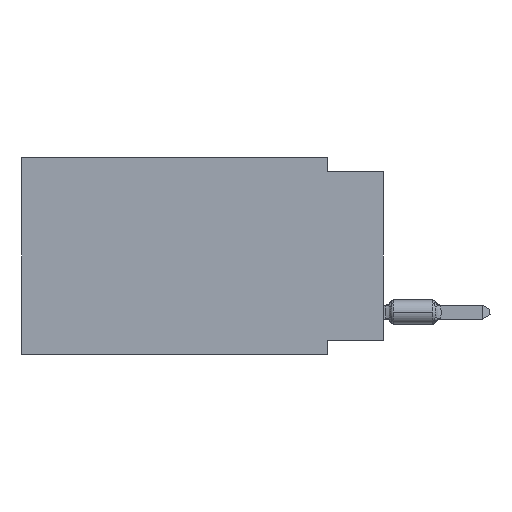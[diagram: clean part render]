
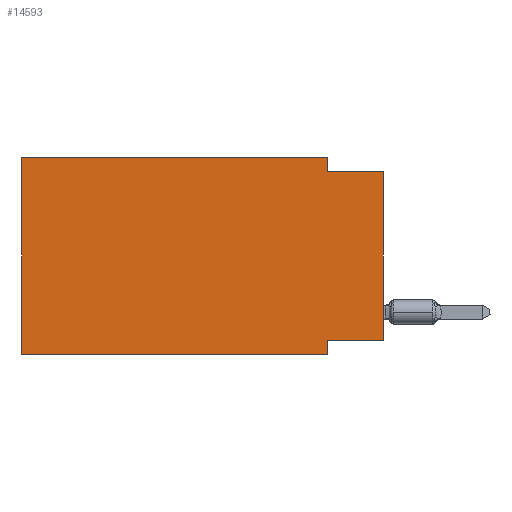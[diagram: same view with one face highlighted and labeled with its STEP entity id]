
A CAD part, left-side view. The second image highlights one B-rep face of the part: STEP entity #14593.
In plain terms, the highlighted planar face has unit normal (-1, 0, 0).
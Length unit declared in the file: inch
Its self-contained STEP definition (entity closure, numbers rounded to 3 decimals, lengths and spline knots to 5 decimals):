
#57 = LINE ( 'NONE', #17755, #11710 ) ;
#176 = CARTESIAN_POINT ( 'NONE',  ( 0., 0., -0.025 ) ) ;
#283 = LINE ( 'NONE', #176, #20078 ) ;
#619 = VERTEX_POINT ( 'NONE', #20172 ) ;
#1433 = EDGE_CURVE ( 'NONE', #3053, #3446, #9642, .T. ) ;
#1984 = CARTESIAN_POINT ( 'NONE',  ( 0., 0.645, 0. ) ) ;
#2115 = VECTOR ( 'NONE', #2336, 39.37008 ) ;
#2336 = DIRECTION ( 'NONE',  ( 0., 1., 0. ) ) ;
#2462 = VERTEX_POINT ( 'NONE', #4624 ) ;
#2981 = DIRECTION ( 'NONE',  ( 0., -1., 0. ) ) ;
#3053 = VERTEX_POINT ( 'NONE', #13976 ) ;
#3055 = LINE ( 'NONE', #16141, #8898 ) ;
#3446 = VERTEX_POINT ( 'NONE', #13425 ) ;
#3547 = EDGE_CURVE ( 'NONE', #9987, #4211, #10963, .T. ) ;
#3903 = LINE ( 'NONE', #1984, #10249 ) ;
#4211 = VERTEX_POINT ( 'NONE', #7042 ) ;
#4624 = CARTESIAN_POINT ( 'NONE',  ( 0., 0.645, 0. ) ) ;
#4730 = VERTEX_POINT ( 'NONE', #16098 ) ;
#5126 = LINE ( 'NONE', #11673, #11326 ) ;
#5226 = DIRECTION ( 'NONE',  ( 0., 0., 1. ) ) ;
#5885 = EDGE_CURVE ( 'NONE', #619, #2462, #3903, .T. ) ;
#5891 = DIRECTION ( 'NONE',  ( 0., 0., -1. ) ) ;
#5955 = ORIENTED_EDGE ( 'NONE', *, *, #10962, .F. ) ;
#6203 = EDGE_CURVE ( 'NONE', #4730, #19444, #3055, .T. ) ;
#6602 = DIRECTION ( 'NONE',  ( 0., -1., 0. ) ) ;
#7042 = CARTESIAN_POINT ( 'NONE',  ( 0., 0., -0.025 ) ) ;
#7087 = EDGE_CURVE ( 'NONE', #619, #3446, #5126, .T. ) ;
#7169 = LINE ( 'NONE', #20258, #2115 ) ;
#7699 = ORIENTED_EDGE ( 'NONE', *, *, #1433, .F. ) ;
#8097 = CARTESIAN_POINT ( 'NONE',  ( 0., 0.1, -0.025 ) ) ;
#8594 = EDGE_CURVE ( 'NONE', #2462, #4730, #57, .T. ) ;
#8715 = ORIENTED_EDGE ( 'NONE', *, *, #8594, .F. ) ;
#8898 = VECTOR ( 'NONE', #9385, 39.37008 ) ;
#9069 = ORIENTED_EDGE ( 'NONE', *, *, #3547, .T. ) ;
#9385 = DIRECTION ( 'NONE',  ( 0., 0., -1. ) ) ;
#9435 = AXIS2_PLACEMENT_3D ( 'NONE', #15853, #11051, #5891 ) ;
#9642 = LINE ( 'NONE', #14679, #19142 ) ;
#9987 = VERTEX_POINT ( 'NONE', #13252 ) ;
#10249 = VECTOR ( 'NONE', #5226, 39.37008 ) ;
#10962 = EDGE_CURVE ( 'NONE', #9987, #3053, #7169, .T. ) ;
#10963 = LINE ( 'NONE', #15668, #15646 ) ;
#11051 = DIRECTION ( 'NONE',  ( 1., 0., 0. ) ) ;
#11326 = VECTOR ( 'NONE', #2981, 39.37008 ) ;
#11673 = CARTESIAN_POINT ( 'NONE',  ( 0., 0.645, -0.35 ) ) ;
#11710 = VECTOR ( 'NONE', #6602, 39.37008 ) ;
#11717 = ORIENTED_EDGE ( 'NONE', *, *, #5885, .F. ) ;
#11982 = ORIENTED_EDGE ( 'NONE', *, *, #20088, .F. ) ;
#12436 = PLANE ( 'NONE',  #9435 ) ;
#13155 = DIRECTION ( 'NONE',  ( 0., -1., 0. ) ) ;
#13252 = CARTESIAN_POINT ( 'NONE',  ( 0., 0., -0.325 ) ) ;
#13281 = DIRECTION ( 'NONE',  ( 0., 0., -1. ) ) ;
#13425 = CARTESIAN_POINT ( 'NONE',  ( 0., 0.1, -0.35 ) ) ;
#13976 = CARTESIAN_POINT ( 'NONE',  ( 0., 0.1, -0.325 ) ) ;
#14593 = ADVANCED_FACE ( 'NONE', ( #20903 ), #12436, .F. ) ;
#14679 = CARTESIAN_POINT ( 'NONE',  ( 0., 0.1, -0.35 ) ) ;
#15624 = ORIENTED_EDGE ( 'NONE', *, *, #6203, .F. ) ;
#15646 = VECTOR ( 'NONE', #20598, 39.37008 ) ;
#15668 = CARTESIAN_POINT ( 'NONE',  ( 0., 0., 0. ) ) ;
#15853 = CARTESIAN_POINT ( 'NONE',  ( 0., 0.645, 0. ) ) ;
#16098 = CARTESIAN_POINT ( 'NONE',  ( 0., 0.1, 0. ) ) ;
#16141 = CARTESIAN_POINT ( 'NONE',  ( 0., 0.1, 0. ) ) ;
#17755 = CARTESIAN_POINT ( 'NONE',  ( 0., 0.645, 0. ) ) ;
#19142 = VECTOR ( 'NONE', #13281, 39.37008 ) ;
#19444 = VERTEX_POINT ( 'NONE', #8097 ) ;
#20078 = VECTOR ( 'NONE', #13155, 39.37008 ) ;
#20088 = EDGE_CURVE ( 'NONE', #19444, #4211, #283, .T. ) ;
#20102 = ORIENTED_EDGE ( 'NONE', *, *, #7087, .T. ) ;
#20172 = CARTESIAN_POINT ( 'NONE',  ( 0., 0.645, -0.35 ) ) ;
#20258 = CARTESIAN_POINT ( 'NONE',  ( 0., 0., -0.325 ) ) ;
#20564 = EDGE_LOOP ( 'NONE', ( #9069, #11982, #15624, #8715, #11717, #20102, #7699, #5955 ) ) ;
#20598 = DIRECTION ( 'NONE',  ( 0., 0., 1. ) ) ;
#20903 = FACE_OUTER_BOUND ( 'NONE', #20564, .T. ) ;
